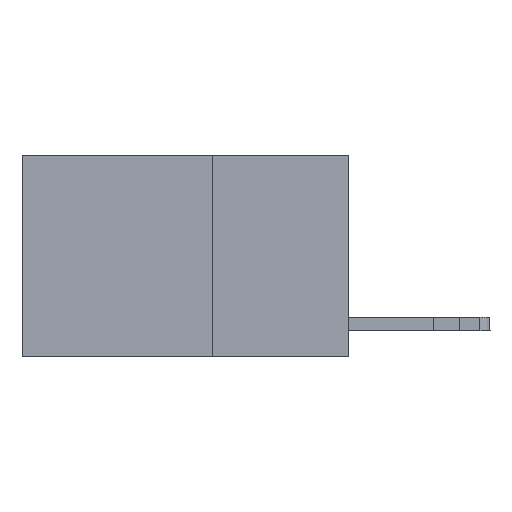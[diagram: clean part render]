
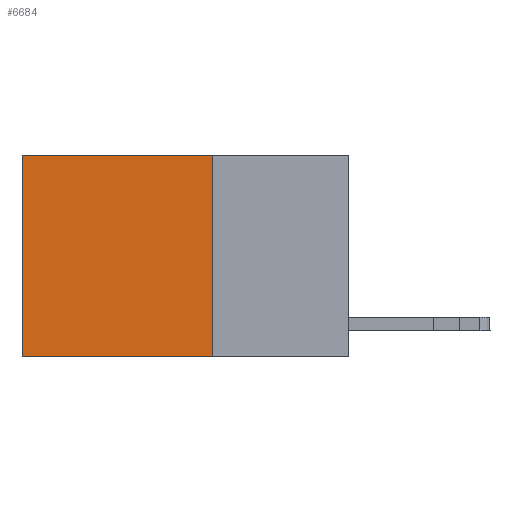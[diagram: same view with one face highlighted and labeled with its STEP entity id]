
A CAD part, left-side view. The second image highlights one B-rep face of the part: STEP entity #6684.
In plain terms, the highlighted planar face has unit normal (-1, 0, 0).
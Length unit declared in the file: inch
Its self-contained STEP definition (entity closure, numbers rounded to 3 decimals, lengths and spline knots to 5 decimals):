
#113 = VECTOR ( 'NONE', #7851, 39.37008 ) ;
#2052 = ORIENTED_EDGE ( 'NONE', *, *, #6105, .T. ) ;
#2685 = LINE ( 'NONE', #22346, #20629 ) ;
#4448 = CARTESIAN_POINT ( 'NONE',  ( 0.2625, 0.6, 0. ) ) ;
#4861 = FACE_OUTER_BOUND ( 'NONE', #5973, .T. ) ;
#5115 = CARTESIAN_POINT ( 'NONE',  ( 0.2625, 0.6, 0. ) ) ;
#5956 = DIRECTION ( 'NONE',  ( 0., 0., -1. ) ) ;
#5973 = EDGE_LOOP ( 'NONE', ( #19809, #20495, #17815, #2052 ) ) ;
#6105 = EDGE_CURVE ( 'NONE', #14086, #8625, #17291, .T. ) ;
#6110 = LINE ( 'NONE', #9590, #113 ) ;
#6266 = VECTOR ( 'NONE', #13522, 39.37008 ) ;
#6447 = CARTESIAN_POINT ( 'NONE',  ( 0.2625, 0.25, 0. ) ) ;
#6502 = DIRECTION ( 'NONE',  ( 0., 0., -1. ) ) ;
#6684 = ADVANCED_FACE ( 'NONE', ( #4861 ), #8135, .F. ) ;
#7119 = CARTESIAN_POINT ( 'NONE',  ( 0.2625, 0.25, -0.37 ) ) ;
#7568 = VECTOR ( 'NONE', #22458, 39.37008 ) ;
#7851 = DIRECTION ( 'NONE',  ( 0., 1., 0. ) ) ;
#8135 = PLANE ( 'NONE',  #22731 ) ;
#8625 = VERTEX_POINT ( 'NONE', #4448 ) ;
#9590 = CARTESIAN_POINT ( 'NONE',  ( 0.2625, 0.25, -0.37 ) ) ;
#10762 = VERTEX_POINT ( 'NONE', #7119 ) ;
#11412 = VERTEX_POINT ( 'NONE', #19572 ) ;
#12917 = EDGE_CURVE ( 'NONE', #14086, #10762, #2685, .T. ) ;
#13522 = DIRECTION ( 'NONE',  ( 0., 1., 0. ) ) ;
#13801 = CARTESIAN_POINT ( 'NONE',  ( 0.2625, 0.25, 0. ) ) ;
#14086 = VERTEX_POINT ( 'NONE', #13801 ) ;
#14871 = EDGE_CURVE ( 'NONE', #8625, #11412, #19162, .T. ) ;
#15331 = DIRECTION ( 'NONE',  ( 1., 0., 0. ) ) ;
#15438 = CARTESIAN_POINT ( 'NONE',  ( 0.2625, 0.25, 0. ) ) ;
#17291 = LINE ( 'NONE', #6447, #6266 ) ;
#17815 = ORIENTED_EDGE ( 'NONE', *, *, #12917, .F. ) ;
#18811 = EDGE_CURVE ( 'NONE', #10762, #11412, #6110, .T. ) ;
#19162 = LINE ( 'NONE', #5115, #7568 ) ;
#19572 = CARTESIAN_POINT ( 'NONE',  ( 0.2625, 0.6, -0.37 ) ) ;
#19809 = ORIENTED_EDGE ( 'NONE', *, *, #14871, .T. ) ;
#20495 = ORIENTED_EDGE ( 'NONE', *, *, #18811, .F. ) ;
#20629 = VECTOR ( 'NONE', #5956, 39.37008 ) ;
#22346 = CARTESIAN_POINT ( 'NONE',  ( 0.2625, 0.25, 0. ) ) ;
#22458 = DIRECTION ( 'NONE',  ( 0., 0., -1. ) ) ;
#22731 = AXIS2_PLACEMENT_3D ( 'NONE', #15438, #15331, #6502 ) ;
